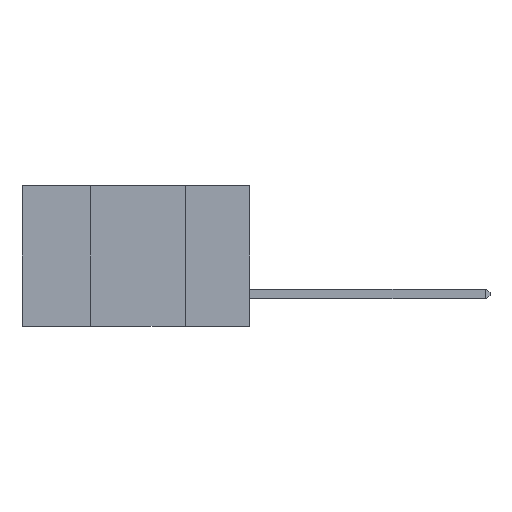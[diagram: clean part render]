
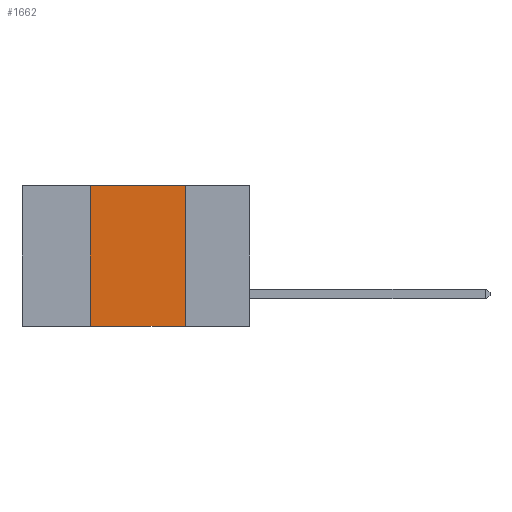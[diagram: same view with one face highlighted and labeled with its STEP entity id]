
A CAD part, left-side view. The second image highlights one B-rep face of the part: STEP entity #1662.
In plain terms, the highlighted planar face has unit normal (-1, 0, 0).
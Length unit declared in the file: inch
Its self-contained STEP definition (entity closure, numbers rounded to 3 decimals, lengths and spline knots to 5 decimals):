
#25 = DIRECTION ( 'NONE',  ( 0., 0., -1. ) ) ;
#476 = VERTEX_POINT ( 'NONE', #4833 ) ;
#755 = DIRECTION ( 'NONE',  ( 0., -1., 0. ) ) ;
#1101 = EDGE_CURVE ( 'NONE', #2545, #476, #13117, .T. ) ;
#1398 = AXIS2_PLACEMENT_3D ( 'NONE', #12914, #6812, #25 ) ;
#1662 = ADVANCED_FACE ( 'NONE', ( #9559 ), #5652, .F. ) ;
#1805 = VECTOR ( 'NONE', #755, 39.37008 ) ;
#2145 = EDGE_CURVE ( 'NONE', #3603, #6116, #5741, .T. ) ;
#2545 = VERTEX_POINT ( 'NONE', #11606 ) ;
#2555 = EDGE_CURVE ( 'NONE', #2545, #6116, #9596, .T. ) ;
#2648 = DIRECTION ( 'NONE',  ( 0., -1., 0. ) ) ;
#2701 = VECTOR ( 'NONE', #10072, 39.37008 ) ;
#3603 = VERTEX_POINT ( 'NONE', #10134 ) ;
#4383 = VECTOR ( 'NONE', #2648, 39.37008 ) ;
#4625 = CARTESIAN_POINT ( 'NONE',  ( 0., 0.17, 0. ) ) ;
#4730 = LINE ( 'NONE', #10312, #4383 ) ;
#4833 = CARTESIAN_POINT ( 'NONE',  ( 0., 0.42, 0. ) ) ;
#5652 = PLANE ( 'NONE',  #1398 ) ;
#5741 = LINE ( 'NONE', #4625, #2701 ) ;
#6116 = VERTEX_POINT ( 'NONE', #13742 ) ;
#6311 = EDGE_CURVE ( 'NONE', #476, #3603, #4730, .T. ) ;
#6812 = DIRECTION ( 'NONE',  ( 1., 0., 0. ) ) ;
#6875 = ORIENTED_EDGE ( 'NONE', *, *, #1101, .F. ) ;
#6997 = EDGE_LOOP ( 'NONE', ( #7919, #10011, #6875, #13361 ) ) ;
#7505 = DIRECTION ( 'NONE',  ( 0., 0., 1. ) ) ;
#7802 = VECTOR ( 'NONE', #7505, 39.37008 ) ;
#7919 = ORIENTED_EDGE ( 'NONE', *, *, #2145, .F. ) ;
#8909 = CARTESIAN_POINT ( 'NONE',  ( 0., 0.42, 0. ) ) ;
#9559 = FACE_OUTER_BOUND ( 'NONE', #6997, .T. ) ;
#9596 = LINE ( 'NONE', #13508, #1805 ) ;
#10011 = ORIENTED_EDGE ( 'NONE', *, *, #6311, .F. ) ;
#10072 = DIRECTION ( 'NONE',  ( 0., 0., -1. ) ) ;
#10134 = CARTESIAN_POINT ( 'NONE',  ( 0., 0.17, 0. ) ) ;
#10312 = CARTESIAN_POINT ( 'NONE',  ( 0., 0.6, 0. ) ) ;
#11606 = CARTESIAN_POINT ( 'NONE',  ( 0., 0.42, -0.37 ) ) ;
#12914 = CARTESIAN_POINT ( 'NONE',  ( 0., 0.6, 0. ) ) ;
#13117 = LINE ( 'NONE', #8909, #7802 ) ;
#13361 = ORIENTED_EDGE ( 'NONE', *, *, #2555, .T. ) ;
#13508 = CARTESIAN_POINT ( 'NONE',  ( 0., 0.6, -0.37 ) ) ;
#13742 = CARTESIAN_POINT ( 'NONE',  ( 0., 0.17, -0.37 ) ) ;
